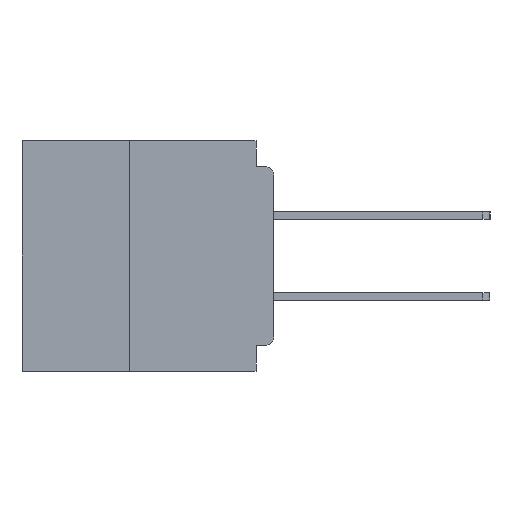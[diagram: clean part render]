
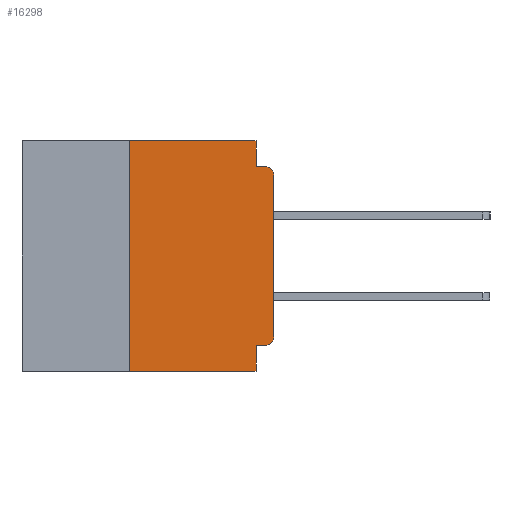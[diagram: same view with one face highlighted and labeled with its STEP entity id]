
A CAD part, left-side view. The second image highlights one B-rep face of the part: STEP entity #16298.
In plain terms, the highlighted planar face has unit normal (-1, 0, 0).
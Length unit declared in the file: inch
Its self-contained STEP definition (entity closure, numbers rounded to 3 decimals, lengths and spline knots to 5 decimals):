
#196 = VECTOR ( 'NONE', #25830, 39.37008 ) ;
#601 = ORIENTED_EDGE ( 'NONE', *, *, #35842, .F. ) ;
#1017 = EDGE_CURVE ( 'NONE', #40671, #3433, #37312, .T. ) ;
#1075 = ORIENTED_EDGE ( 'NONE', *, *, #7718, .F. ) ;
#1348 = DIRECTION ( 'NONE',  ( 0., 0., -1. ) ) ;
#1409 = DIRECTION ( 'NONE',  ( 0., -1., 0. ) ) ;
#1520 = ORIENTED_EDGE ( 'NONE', *, *, #15549, .F. ) ;
#1636 = LINE ( 'NONE', #36461, #37989 ) ;
#3102 = VECTOR ( 'NONE', #1409, 39.37008 ) ;
#3433 = VERTEX_POINT ( 'NONE', #43321 ) ;
#3651 = EDGE_CURVE ( 'NONE', #23839, #16164, #30585, .T. ) ;
#4233 = LINE ( 'NONE', #29629, #3102 ) ;
#4326 = ORIENTED_EDGE ( 'NONE', *, *, #32122, .F. ) ;
#4355 = VECTOR ( 'NONE', #13921, 39.37008 ) ;
#5376 = ORIENTED_EDGE ( 'NONE', *, *, #14796, .T. ) ;
#5839 = LINE ( 'NONE', #32271, #31716 ) ;
#5843 = VERTEX_POINT ( 'NONE', #34187 ) ;
#5960 = ORIENTED_EDGE ( 'NONE', *, *, #19842, .T. ) ;
#7294 = CARTESIAN_POINT ( 'NONE',  ( 0., 0.031, -0.4 ) ) ;
#7718 = EDGE_CURVE ( 'NONE', #23839, #15019, #32431, .T. ) ;
#7757 = VERTEX_POINT ( 'NONE', #35082 ) ;
#8430 = CARTESIAN_POINT ( 'NONE',  ( 0., 0.25, -0.4 ) ) ;
#8931 = VERTEX_POINT ( 'NONE', #27994 ) ;
#10799 = DIRECTION ( 'NONE',  ( 0., 0., -1. ) ) ;
#11332 = DIRECTION ( 'NONE',  ( 0., -1., 0. ) ) ;
#12054 = ORIENTED_EDGE ( 'NONE', *, *, #1017, .T. ) ;
#12220 = DIRECTION ( 'NONE',  ( -1., 0., 0. ) ) ;
#13921 = DIRECTION ( 'NONE',  ( 0., 0., 1. ) ) ;
#14796 = EDGE_CURVE ( 'NONE', #7757, #40671, #44882, .T. ) ;
#14874 = LINE ( 'NONE', #25034, #32476 ) ;
#15019 = VERTEX_POINT ( 'NONE', #29855 ) ;
#15462 = CARTESIAN_POINT ( 'NONE',  ( 0., 0.437, 0. ) ) ;
#15549 = EDGE_CURVE ( 'NONE', #8931, #3433, #5839, .T. ) ;
#16164 = VERTEX_POINT ( 'NONE', #18249 ) ;
#16298 = ADVANCED_FACE ( 'NONE', ( #19597 ), #36502, .F. ) ;
#16451 = AXIS2_PLACEMENT_3D ( 'NONE', #33285, #12220, #36825 ) ;
#16622 = ORIENTED_EDGE ( 'NONE', *, *, #3651, .T. ) ;
#17753 = CIRCLE ( 'NONE', #20692, 0.015 ) ;
#17854 = DIRECTION ( 'NONE',  ( -1., 0., 0. ) ) ;
#18038 = VECTOR ( 'NONE', #28618, 39.37008 ) ;
#18249 = CARTESIAN_POINT ( 'NONE',  ( 0., 0.031, -0.4 ) ) ;
#19023 = DIRECTION ( 'NONE',  ( 0., 0., -1. ) ) ;
#19313 = CARTESIAN_POINT ( 'NONE',  ( 0., 0.031, 0. ) ) ;
#19597 = FACE_OUTER_BOUND ( 'NONE', #45164, .T. ) ;
#19842 = EDGE_CURVE ( 'NONE', #39345, #7757, #17753, .T. ) ;
#20692 = AXIS2_PLACEMENT_3D ( 'NONE', #38857, #17854, #42350 ) ;
#21626 = CARTESIAN_POINT ( 'NONE',  ( 0., 0., 0. ) ) ;
#23839 = VERTEX_POINT ( 'NONE', #8430 ) ;
#23931 = ORIENTED_EDGE ( 'NONE', *, *, #39410, .F. ) ;
#25034 = CARTESIAN_POINT ( 'NONE',  ( 0., 0., -0.355 ) ) ;
#25669 = ORIENTED_EDGE ( 'NONE', *, *, #45534, .F. ) ;
#25830 = DIRECTION ( 'NONE',  ( 0., -1., 0. ) ) ;
#27994 = CARTESIAN_POINT ( 'NONE',  ( 0., 0.031, -0.045 ) ) ;
#28525 = DIRECTION ( 'NONE',  ( 0., 1., 0. ) ) ;
#28618 = DIRECTION ( 'NONE',  ( 0., 0., 1. ) ) ;
#29332 = CARTESIAN_POINT ( 'NONE',  ( 0., 0.015, -0.355 ) ) ;
#29629 = CARTESIAN_POINT ( 'NONE',  ( 0., 0.437, 0. ) ) ;
#29855 = CARTESIAN_POINT ( 'NONE',  ( 0., 0.25, 0. ) ) ;
#30585 = LINE ( 'NONE', #39731, #196 ) ;
#31716 = VECTOR ( 'NONE', #11332, 39.37008 ) ;
#32122 = EDGE_CURVE ( 'NONE', #39345, #5843, #14874, .T. ) ;
#32271 = CARTESIAN_POINT ( 'NONE',  ( 0., 0., -0.045 ) ) ;
#32431 = LINE ( 'NONE', #34937, #4355 ) ;
#32476 = VECTOR ( 'NONE', #28525, 39.37008 ) ;
#33285 = CARTESIAN_POINT ( 'NONE',  ( 0., 0.015, -0.06 ) ) ;
#33456 = AXIS2_PLACEMENT_3D ( 'NONE', #15462, #40009, #19023 ) ;
#34187 = CARTESIAN_POINT ( 'NONE',  ( 0., 0.031, -0.355 ) ) ;
#34937 = CARTESIAN_POINT ( 'NONE',  ( 0., 0.25, -0.4 ) ) ;
#35082 = CARTESIAN_POINT ( 'NONE',  ( 0., 0., -0.34 ) ) ;
#35842 = EDGE_CURVE ( 'NONE', #5843, #16164, #41921, .T. ) ;
#36461 = CARTESIAN_POINT ( 'NONE',  ( 0., 0.031, 0. ) ) ;
#36502 = PLANE ( 'NONE',  #33456 ) ;
#36825 = DIRECTION ( 'NONE',  ( 0., 0., -1. ) ) ;
#37312 = CIRCLE ( 'NONE', #16451, 0.015 ) ;
#37989 = VECTOR ( 'NONE', #1348, 39.37008 ) ;
#38857 = CARTESIAN_POINT ( 'NONE',  ( 0., 0.015, -0.34 ) ) ;
#39345 = VERTEX_POINT ( 'NONE', #29332 ) ;
#39410 = EDGE_CURVE ( 'NONE', #15019, #41346, #4233, .T. ) ;
#39731 = CARTESIAN_POINT ( 'NONE',  ( 0., 0.437, -0.4 ) ) ;
#39926 = CARTESIAN_POINT ( 'NONE',  ( 0., 0., -0.06 ) ) ;
#40009 = DIRECTION ( 'NONE',  ( 1., 0., 0. ) ) ;
#40671 = VERTEX_POINT ( 'NONE', #39926 ) ;
#40852 = VECTOR ( 'NONE', #10799, 39.37008 ) ;
#41346 = VERTEX_POINT ( 'NONE', #19313 ) ;
#41921 = LINE ( 'NONE', #7294, #40852 ) ;
#42350 = DIRECTION ( 'NONE',  ( 0., 0., -1. ) ) ;
#43321 = CARTESIAN_POINT ( 'NONE',  ( 0., 0.015, -0.045 ) ) ;
#44882 = LINE ( 'NONE', #21626, #18038 ) ;
#45164 = EDGE_LOOP ( 'NONE', ( #5376, #12054, #1520, #25669, #23931, #1075, #16622, #601, #4326, #5960 ) ) ;
#45534 = EDGE_CURVE ( 'NONE', #41346, #8931, #1636, .T. ) ;
